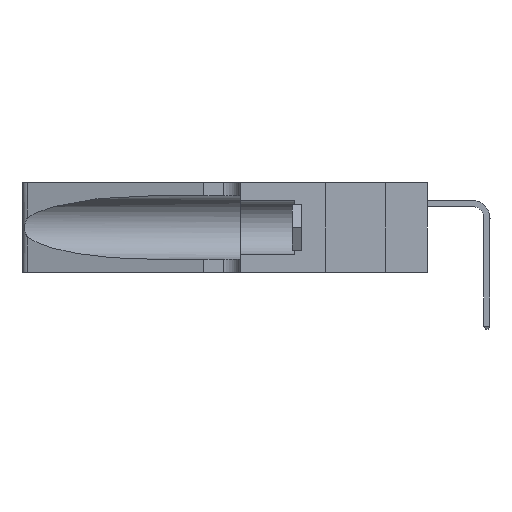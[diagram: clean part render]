
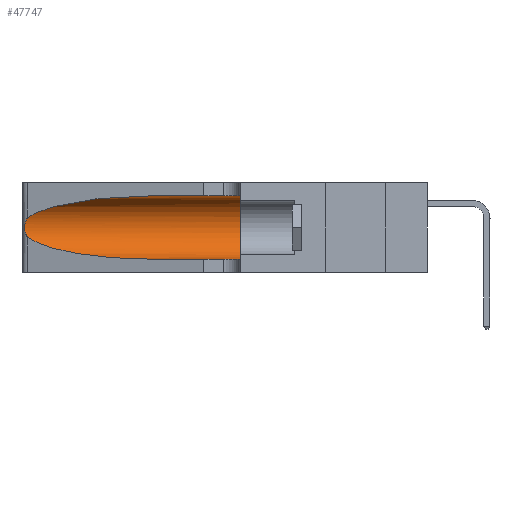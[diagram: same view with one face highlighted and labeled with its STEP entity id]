
A CAD part, left-side view. The second image highlights one B-rep face of the part: STEP entity #47747.
In plain terms, the highlighted cylindrical face has radius 3.308 mm (diameter 6.617 mm), a partial arc.
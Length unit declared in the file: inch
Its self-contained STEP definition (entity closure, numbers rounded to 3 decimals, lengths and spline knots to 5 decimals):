
#28 = CARTESIAN_POINT ( 'NONE',  ( 0.25856, 1.23593, 0.16098 ) ) ;
#172 = EDGE_LOOP ( 'NONE', ( #8500, #23029, #24951, #7321, #42842, #35816 ) ) ;
#3033 = CARTESIAN_POINT ( 'NONE',  ( 0.18966, 0.96281, 0.31525 ) ) ;
#3182 = EDGE_CURVE ( 'NONE', #41464, #43674, #15071, .T. ) ;
#3349 = VECTOR ( 'NONE', #26932, 39.37008 ) ;
#3633 = CARTESIAN_POINT ( 'NONE',  ( 0.2373, 1.15595, 0.08982 ) ) ;
#4101 = CARTESIAN_POINT ( 'NONE',  ( 0.25639, 1.23186, 0.15144 ) ) ;
#7321 = ORIENTED_EDGE ( 'NONE', *, *, #3182, .T. ) ;
#7696 = CARTESIAN_POINT ( 'NONE',  ( 0.18966, 0.96281, 0.05475 ) ) ;
#8155 = CARTESIAN_POINT ( 'NONE',  ( 0.25487, 1.22718, 0.14631 ) ) ;
#8338 = CARTESIAN_POINT ( 'NONE',  ( 0.1305, 0.72297, 0.31525 ) ) ;
#8500 = ORIENTED_EDGE ( 'NONE', *, *, #16537, .T. ) ;
#10684 = CARTESIAN_POINT ( 'NONE',  ( 0.25487, 1.22718, 0.22369 ) ) ;
#10950 = CARTESIAN_POINT ( 'NONE',  ( 0.1305, 0.35, 0.31525 ) ) ;
#11141 = CARTESIAN_POINT ( 'NONE',  ( 0.1305, 0.72297, 0.31525 ) ) ;
#12056 = CARTESIAN_POINT ( 'NONE',  ( 0.25639, 1.23184, 0.21858 ) ) ;
#12097 = FACE_OUTER_BOUND ( 'NONE', #172, .T. ) ;
#14745 = VERTEX_POINT ( 'NONE', #10950 ) ;
#15071 = LINE ( 'NONE', #19394, #35308 ) ;
#15347 = DIRECTION ( 'NONE',  ( 0., -1., 0. ) ) ;
#16107 = CARTESIAN_POINT ( 'NONE',  ( 0.25854, 1.2359, 0.20912 ) ) ;
#16469 = CIRCLE ( 'NONE', #29479, 0.13025 ) ;
#16537 = EDGE_CURVE ( 'NONE', #29360, #47751, #48850, .T. ) ;
#16992 = EDGE_CURVE ( 'NONE', #29360, #14745, #35603, .T. ) ;
#18156 = AXIS2_PLACEMENT_3D ( 'NONE', #51105, #26718, #30777 ) ;
#18814 = CARTESIAN_POINT ( 'NONE',  ( 0.1305, 1.61858, 0.31525 ) ) ;
#19002 = CARTESIAN_POINT ( 'NONE',  ( 0.1305, 0.35, 0.185 ) ) ;
#19394 = CARTESIAN_POINT ( 'NONE',  ( 0.1305, 1.61858, 0.05475 ) ) ;
#20194 = CARTESIAN_POINT ( 'NONE',  ( 0.26075, 1.23896, 0.19203 ) ) ;
#21518 = CARTESIAN_POINT ( 'NONE',  ( 0.1305, 0.72297, 0.05475 ) ) ;
#23029 = ORIENTED_EDGE ( 'NONE', *, *, #47966, .T. ) ;
#23040 = DIRECTION ( 'NONE',  ( 0., 0., 1. ) ) ;
#24201 = CARTESIAN_POINT ( 'NONE',  ( 0.26017, 1.23833, 0.17102 ) ) ;
#24951 = ORIENTED_EDGE ( 'NONE', *, *, #51076, .T. ) ;
#26718 = DIRECTION ( 'NONE',  ( 0., -1., 0. ) ) ;
#26932 = DIRECTION ( 'NONE',  ( 0., -1., 0. ) ) ;
#28087 = CARTESIAN_POINT ( 'NONE',  ( 0.25555, 1.22994, 0.2215 ) ) ;
#28263 = CARTESIAN_POINT ( 'NONE',  ( 0.25789, 1.23486, 0.15765 ) ) ;
#29360 = VERTEX_POINT ( 'NONE', #8338 ) ;
#29479 = AXIS2_PLACEMENT_3D ( 'NONE', #19002, #47413, #23040 ) ;
#30777 = DIRECTION ( 'NONE',  ( 0., 0., -1. ) ) ;
#30954 = B_SPLINE_CURVE_WITH_KNOTS ( 'NONE', 3,
 ( #36104, #28087, #12056, #40409, #16107, #44487, #20194, #48591, #24201, #28, #28263, #4101, #32375, #8155 ),
 .UNSPECIFIED., .F., .F.,
 ( 4, 2, 2, 2, 2, 2, 4 ),
 ( 0., 0.00027, 0.00053, 0.00107, 0.0016, 0.00187, 0.00214 ),
 .UNSPECIFIED. ) ;
#32375 = CARTESIAN_POINT ( 'NONE',  ( 0.25555, 1.22993, 0.14849 ) ) ;
#35308 = VECTOR ( 'NONE', #15347, 39.37008 ) ;
#35603 = LINE ( 'NONE', #18814, #3349 ) ;
#35816 = ORIENTED_EDGE ( 'NONE', *, *, #16992, .F. ) ;
#35968 = CARTESIAN_POINT ( 'NONE',  ( 0.1305, 0.72297, 0.05475 ) ) ;
#36104 = CARTESIAN_POINT ( 'NONE',  ( 0.25487, 1.22718, 0.22369 ) ) ;
#37247 =( BOUNDED_CURVE ( )  B_SPLINE_CURVE ( 3, ( #39925, #3633, #7696, #35968 ),
 .UNSPECIFIED., .F., .F. ) 
 B_SPLINE_CURVE_WITH_KNOTS ( ( 4, 4 ),
 ( 3.44316, 4.71239 ),
 .UNSPECIFIED. ) 
 CURVE ( )  GEOMETRIC_REPRESENTATION_ITEM ( )  RATIONAL_B_SPLINE_CURVE ( ( 1., 0.87, 0.87, 1. ) ) 
 REPRESENTATION_ITEM ( '' )  );
#39239 = CARTESIAN_POINT ( 'NONE',  ( 0.1305, 0.35, 0.05475 ) ) ;
#39479 = CARTESIAN_POINT ( 'NONE',  ( 0.25487, 1.22718, 0.22369 ) ) ;
#39925 = CARTESIAN_POINT ( 'NONE',  ( 0.25487, 1.22718, 0.14631 ) ) ;
#40409 = CARTESIAN_POINT ( 'NONE',  ( 0.25787, 1.23484, 0.2124 ) ) ;
#40629 = CYLINDRICAL_SURFACE ( 'NONE', #18156, 0.13025 ) ;
#41464 = VERTEX_POINT ( 'NONE', #21518 ) ;
#42842 = ORIENTED_EDGE ( 'NONE', *, *, #43669, .F. ) ;
#43669 = EDGE_CURVE ( 'NONE', #14745, #43674, #16469, .T. ) ;
#43674 = VERTEX_POINT ( 'NONE', #39239 ) ;
#44176 = CARTESIAN_POINT ( 'NONE',  ( 0.25487, 1.22718, 0.14631 ) ) ;
#44487 = CARTESIAN_POINT ( 'NONE',  ( 0.26018, 1.23835, 0.19895 ) ) ;
#47413 = DIRECTION ( 'NONE',  ( 0., 1., 0. ) ) ;
#47499 = CARTESIAN_POINT ( 'NONE',  ( 0.2373, 1.15595, 0.28018 ) ) ;
#47747 = ADVANCED_FACE ( 'NONE', ( #12097 ), #40629, .F. ) ;
#47751 = VERTEX_POINT ( 'NONE', #10684 ) ;
#47966 = EDGE_CURVE ( 'NONE', #47751, #51079, #30954, .T. ) ;
#48591 = CARTESIAN_POINT ( 'NONE',  ( 0.26075, 1.23896, 0.178 ) ) ;
#48850 =( BOUNDED_CURVE ( )  B_SPLINE_CURVE ( 3, ( #11141, #3033, #47499, #39479 ),
 .UNSPECIFIED., .F., .F. ) 
 B_SPLINE_CURVE_WITH_KNOTS ( ( 4, 4 ),
 ( 1.5708, 2.84003 ),
 .UNSPECIFIED. ) 
 CURVE ( )  GEOMETRIC_REPRESENTATION_ITEM ( )  RATIONAL_B_SPLINE_CURVE ( ( 1., 0.87, 0.87, 1. ) ) 
 REPRESENTATION_ITEM ( '' )  );
#51076 = EDGE_CURVE ( 'NONE', #51079, #41464, #37247, .T. ) ;
#51079 = VERTEX_POINT ( 'NONE', #44176 ) ;
#51105 = CARTESIAN_POINT ( 'NONE',  ( 0.1305, 1.61858, 0.185 ) ) ;
